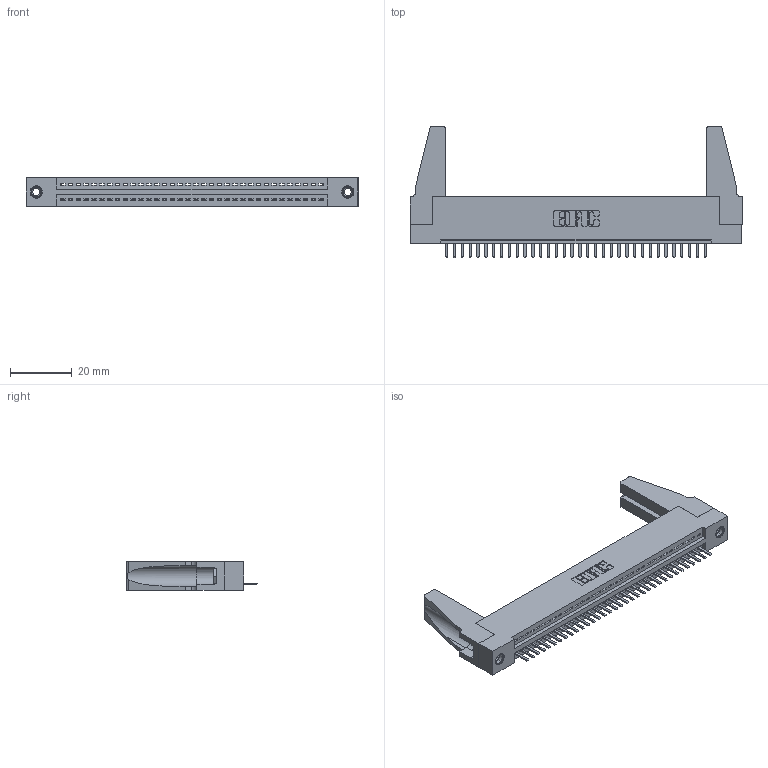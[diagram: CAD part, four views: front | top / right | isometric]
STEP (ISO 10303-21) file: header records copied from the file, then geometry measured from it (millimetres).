
FILE_DESCRIPTION (( 'STEP AP203' ), '1' );
FILE_NAME ('395-034-520-188.STEP', '2019-10-19T16:47:51', ( '' ), ( '' ), 'SwSTEP 2.0', 'SolidWorks 2016', '' );
FILE_SCHEMA (( 'CONFIG_CONTROL_DESIGN' ));
Length unit declared in the file: inch
Products named in the file (5): 345-250-001_345-250-001-102; 345-292-001_345-293-120; 395-034-520-188; 345-220-078_345-220-088; 345 Part_Flush Mounting Lugs - 0.156 Dia-TH
Assembly tree (39 placements, depth 2):
  395-034-520-188
    345 Part_Flush Mounting Lugs - 0.156 Dia-TH
    345-292-001_345-293-120  x34
    345-250-001_345-250-001-102  x2
    345-220-078_345-220-088  x2
Bounding box: 107.59 x 42.55 x 9.4 mm (x, y, z)
Volume: 13308.6 mm3; surface area: 16064.2 mm2
Topology: 39 solids, 39 shells, 2358 faces, 6911 edges, 4506 vertices
Faces by surface type: plane 1580, cylinder 762, cone 12, torus 4
Entity records: 28928 total; most frequent: CARTESIAN_POINT 5012, ORIENTED_EDGE 4928, DIRECTION 4384, EDGE_CURVE 2464, VECTOR 2150, LINE 2150, VERTEX_POINT 1634, AXIS2_PLACEMENT_3D 1117
